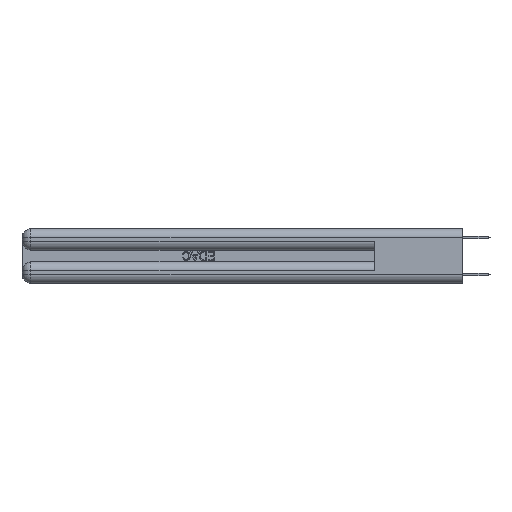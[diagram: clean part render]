
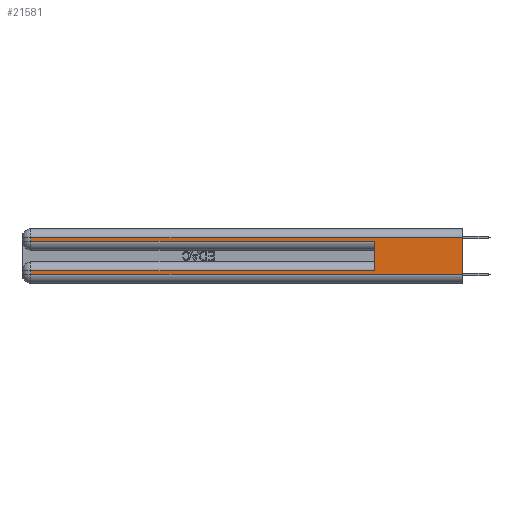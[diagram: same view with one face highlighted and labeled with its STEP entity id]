
A CAD part, left-side view. The second image highlights one B-rep face of the part: STEP entity #21581.
In plain terms, the highlighted planar face has unit normal (-1, 0, 0).
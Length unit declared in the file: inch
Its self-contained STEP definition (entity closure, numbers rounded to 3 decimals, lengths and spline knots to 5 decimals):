
#463 = VECTOR ( 'NONE', #19384, 39.37008 ) ;
#777 = VECTOR ( 'NONE', #13656, 39.37008 ) ;
#1156 = CARTESIAN_POINT ( 'NONE',  ( 0., 0., 0.06 ) ) ;
#2329 = CARTESIAN_POINT ( 'NONE',  ( 0., 0., 0.37 ) ) ;
#2731 = CARTESIAN_POINT ( 'NONE',  ( 0., 2.94, 0.37 ) ) ;
#3383 = ORIENTED_EDGE ( 'NONE', *, *, #27744, .T. ) ;
#3614 = DIRECTION ( 'NONE',  ( 0., 0., -1. ) ) ;
#3649 = VECTOR ( 'NONE', #9351, 39.37008 ) ;
#4139 = VERTEX_POINT ( 'NONE', #22720 ) ;
#4916 = EDGE_CURVE ( 'NONE', #27012, #14180, #7964, .T. ) ;
#5303 = EDGE_CURVE ( 'NONE', #14180, #4139, #27868, .T. ) ;
#5578 = CARTESIAN_POINT ( 'NONE',  ( 0., 0., 0.31 ) ) ;
#6015 = CARTESIAN_POINT ( 'NONE',  ( 0., 2.94, 0.37 ) ) ;
#6032 = VERTEX_POINT ( 'NONE', #10847 ) ;
#6362 = ORIENTED_EDGE ( 'NONE', *, *, #10905, .F. ) ;
#7199 = VECTOR ( 'NONE', #3614, 39.37008 ) ;
#7310 = VERTEX_POINT ( 'NONE', #21144 ) ;
#7571 = EDGE_CURVE ( 'NONE', #6032, #34998, #8827, .T. ) ;
#7574 = ORIENTED_EDGE ( 'NONE', *, *, #23836, .T. ) ;
#7869 = DIRECTION ( 'NONE',  ( 1., 0., 0. ) ) ;
#7964 = LINE ( 'NONE', #5578, #777 ) ;
#8007 = VECTOR ( 'NONE', #20011, 39.37008 ) ;
#8827 = LINE ( 'NONE', #25347, #8007 ) ;
#9351 = DIRECTION ( 'NONE',  ( 0., 0., 1. ) ) ;
#10847 = CARTESIAN_POINT ( 'NONE',  ( 0., 2.94, 0.06 ) ) ;
#10905 = EDGE_CURVE ( 'NONE', #27012, #34998, #30229, .T. ) ;
#10982 = PLANE ( 'NONE',  #33079 ) ;
#11097 = VERTEX_POINT ( 'NONE', #30327 ) ;
#11273 = EDGE_LOOP ( 'NONE', ( #6362, #20113, #27791, #7574, #26766, #3383, #17237, #16400 ) ) ;
#11356 = CARTESIAN_POINT ( 'NONE',  ( 0., 0., 0.37 ) ) ;
#11438 = CARTESIAN_POINT ( 'NONE',  ( 0., 0., 0.31 ) ) ;
#13656 = DIRECTION ( 'NONE',  ( 0., 1., 0. ) ) ;
#13929 = DIRECTION ( 'NONE',  ( 0., 0., -1. ) ) ;
#14180 = VERTEX_POINT ( 'NONE', #17148 ) ;
#16346 = EDGE_CURVE ( 'NONE', #7310, #23612, #28440, .T. ) ;
#16400 = ORIENTED_EDGE ( 'NONE', *, *, #7571, .T. ) ;
#16792 = EDGE_CURVE ( 'NONE', #11097, #6032, #17201, .T. ) ;
#17148 = CARTESIAN_POINT ( 'NONE',  ( 0., 2.94, 0.31 ) ) ;
#17201 = LINE ( 'NONE', #6015, #7199 ) ;
#17237 = ORIENTED_EDGE ( 'NONE', *, *, #16792, .T. ) ;
#19384 = DIRECTION ( 'NONE',  ( 0., 0., -1. ) ) ;
#19596 = FACE_OUTER_BOUND ( 'NONE', #11273, .T. ) ;
#19992 = CARTESIAN_POINT ( 'NONE',  ( 0., 0., 0.285 ) ) ;
#20011 = DIRECTION ( 'NONE',  ( 0., -1., 0. ) ) ;
#20113 = ORIENTED_EDGE ( 'NONE', *, *, #4916, .T. ) ;
#20181 = DIRECTION ( 'NONE',  ( 0., -1., 0. ) ) ;
#20915 = DIRECTION ( 'NONE',  ( 0., 1., 0. ) ) ;
#21144 = CARTESIAN_POINT ( 'NONE',  ( 0., 0.6, 0.085 ) ) ;
#21453 = LINE ( 'NONE', #29340, #31010 ) ;
#21581 = ADVANCED_FACE ( 'NONE', ( #19596 ), #10982, .F. ) ;
#22163 = DIRECTION ( 'NONE',  ( 0., 0., -1. ) ) ;
#22720 = CARTESIAN_POINT ( 'NONE',  ( 0., 2.94, 0.285 ) ) ;
#22751 = CARTESIAN_POINT ( 'NONE',  ( 0., 0.6, 0.145 ) ) ;
#23591 = VECTOR ( 'NONE', #13929, 39.37008 ) ;
#23612 = VERTEX_POINT ( 'NONE', #27711 ) ;
#23836 = EDGE_CURVE ( 'NONE', #4139, #23612, #33792, .T. ) ;
#25347 = CARTESIAN_POINT ( 'NONE',  ( 0., 0., 0.06 ) ) ;
#26766 = ORIENTED_EDGE ( 'NONE', *, *, #16346, .F. ) ;
#27012 = VERTEX_POINT ( 'NONE', #11438 ) ;
#27711 = CARTESIAN_POINT ( 'NONE',  ( 0., 0.6, 0.285 ) ) ;
#27744 = EDGE_CURVE ( 'NONE', #7310, #11097, #21453, .T. ) ;
#27791 = ORIENTED_EDGE ( 'NONE', *, *, #5303, .T. ) ;
#27868 = LINE ( 'NONE', #2731, #23591 ) ;
#28440 = LINE ( 'NONE', #22751, #3649 ) ;
#28494 = VECTOR ( 'NONE', #20181, 39.37008 ) ;
#29340 = CARTESIAN_POINT ( 'NONE',  ( 0., 0., 0.085 ) ) ;
#30229 = LINE ( 'NONE', #2329, #463 ) ;
#30327 = CARTESIAN_POINT ( 'NONE',  ( 0., 2.94, 0.085 ) ) ;
#31010 = VECTOR ( 'NONE', #20915, 39.37008 ) ;
#33079 = AXIS2_PLACEMENT_3D ( 'NONE', #11356, #7869, #22163 ) ;
#33792 = LINE ( 'NONE', #19992, #28494 ) ;
#34998 = VERTEX_POINT ( 'NONE', #1156 ) ;
